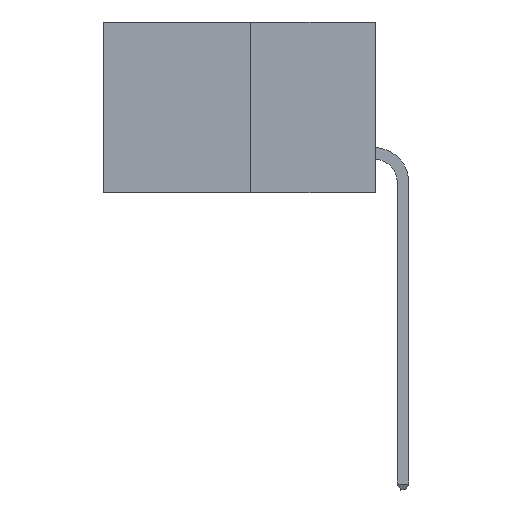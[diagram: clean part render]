
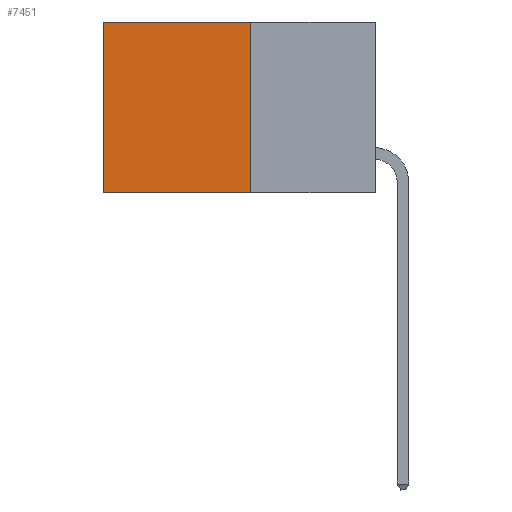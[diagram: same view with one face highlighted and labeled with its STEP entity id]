
A CAD part, left-side view. The second image highlights one B-rep face of the part: STEP entity #7451.
In plain terms, the highlighted planar face has unit normal (-1, 0, 0).
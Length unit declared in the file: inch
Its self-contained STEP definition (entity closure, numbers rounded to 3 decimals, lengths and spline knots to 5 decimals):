
#508 = VERTEX_POINT ( 'NONE', #14061 ) ;
#984 = AXIS2_PLACEMENT_3D ( 'NONE', #1404, #2777, #12407 ) ;
#1404 = CARTESIAN_POINT ( 'NONE',  ( 0.277, 0.27, -0.37 ) ) ;
#1549 = CARTESIAN_POINT ( 'NONE',  ( 0.277, 0.59, -0.37 ) ) ;
#1701 = LINE ( 'NONE', #16252, #15737 ) ;
#2234 = CARTESIAN_POINT ( 'NONE',  ( 0.277, 0.59, -0.37 ) ) ;
#2439 = CARTESIAN_POINT ( 'NONE',  ( 0.277, 0.27, 0. ) ) ;
#2777 = DIRECTION ( 'NONE',  ( 1., 0., 0. ) ) ;
#3736 = VECTOR ( 'NONE', #8464, 39.37008 ) ;
#4174 = LINE ( 'NONE', #1549, #3736 ) ;
#4980 = VERTEX_POINT ( 'NONE', #11256 ) ;
#6859 = DIRECTION ( 'NONE',  ( 0., 1., 0. ) ) ;
#7020 = EDGE_CURVE ( 'NONE', #4980, #508, #12941, .T. ) ;
#7451 = ADVANCED_FACE ( 'NONE', ( #14148 ), #17673, .F. ) ;
#8464 = DIRECTION ( 'NONE',  ( 0., 0., -1. ) ) ;
#8600 = EDGE_CURVE ( 'NONE', #4980, #15739, #10737, .T. ) ;
#8814 = EDGE_LOOP ( 'NONE', ( #11306, #13332, #16892, #14144 ) ) ;
#9413 = VECTOR ( 'NONE', #15493, 39.37008 ) ;
#10737 = LINE ( 'NONE', #2439, #14633 ) ;
#11197 = EDGE_CURVE ( 'NONE', #15739, #16914, #4174, .T. ) ;
#11256 = CARTESIAN_POINT ( 'NONE',  ( 0.277, 0.27, 0. ) ) ;
#11306 = ORIENTED_EDGE ( 'NONE', *, *, #11197, .T. ) ;
#12087 = DIRECTION ( 'NONE',  ( 0., 1., 0. ) ) ;
#12407 = DIRECTION ( 'NONE',  ( 0., 0., -1. ) ) ;
#12775 = CARTESIAN_POINT ( 'NONE',  ( 0.277, 0.27, -0.37 ) ) ;
#12941 = LINE ( 'NONE', #12775, #9413 ) ;
#13191 = EDGE_CURVE ( 'NONE', #508, #16914, #1701, .T. ) ;
#13332 = ORIENTED_EDGE ( 'NONE', *, *, #13191, .F. ) ;
#13494 = CARTESIAN_POINT ( 'NONE',  ( 0.277, 0.59, 0. ) ) ;
#14061 = CARTESIAN_POINT ( 'NONE',  ( 0.277, 0.27, -0.37 ) ) ;
#14144 = ORIENTED_EDGE ( 'NONE', *, *, #8600, .T. ) ;
#14148 = FACE_OUTER_BOUND ( 'NONE', #8814, .T. ) ;
#14633 = VECTOR ( 'NONE', #12087, 39.37008 ) ;
#15493 = DIRECTION ( 'NONE',  ( 0., 0., -1. ) ) ;
#15737 = VECTOR ( 'NONE', #6859, 39.37008 ) ;
#15739 = VERTEX_POINT ( 'NONE', #13494 ) ;
#16252 = CARTESIAN_POINT ( 'NONE',  ( 0.277, 0.27, -0.37 ) ) ;
#16892 = ORIENTED_EDGE ( 'NONE', *, *, #7020, .F. ) ;
#16914 = VERTEX_POINT ( 'NONE', #2234 ) ;
#17673 = PLANE ( 'NONE',  #984 ) ;
